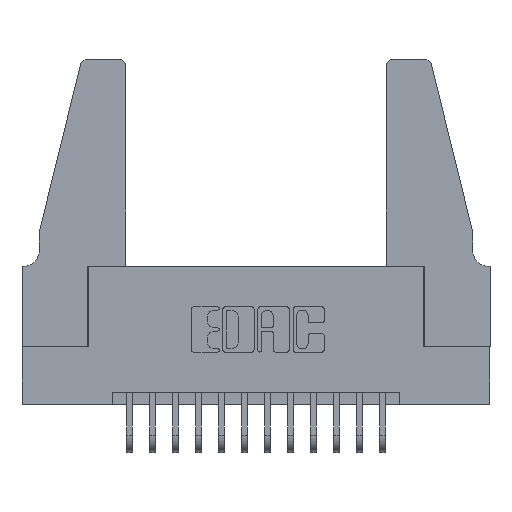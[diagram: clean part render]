
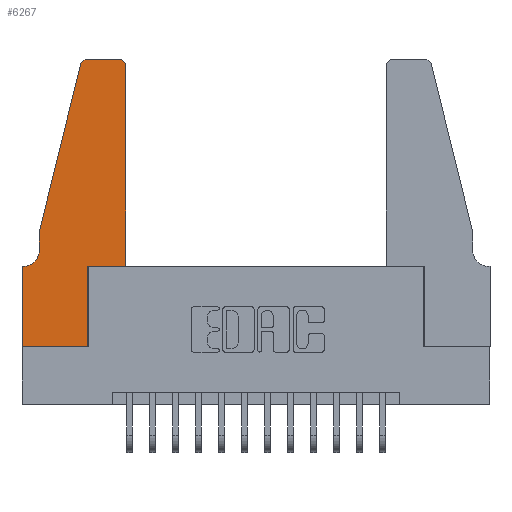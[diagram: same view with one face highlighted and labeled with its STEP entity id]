
A CAD part, top view. The second image highlights one B-rep face of the part: STEP entity #6267.
In plain terms, the highlighted planar face has unit normal (0, 0, 1).
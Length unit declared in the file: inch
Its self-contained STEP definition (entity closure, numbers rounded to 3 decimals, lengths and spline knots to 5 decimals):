
#64 = CARTESIAN_POINT ( 'NONE',  ( 0.2865, 0., 0.37 ) ) ;
#475 = LINE ( 'NONE', #2888, #3563 ) ;
#807 = LINE ( 'NONE', #5140, #5174 ) ;
#1021 = CARTESIAN_POINT ( 'NONE',  ( 0., 0.35, 0.37 ) ) ;
#1147 = EDGE_CURVE ( 'NONE', #10540, #1891, #5495, .T. ) ;
#1408 = CARTESIAN_POINT ( 'NONE',  ( 0.4205, 1.22, 0.37 ) ) ;
#1547 = LINE ( 'NONE', #10497, #8268 ) ;
#1662 = PLANE ( 'NONE',  #8798 ) ;
#1831 = CARTESIAN_POINT ( 'NONE',  ( 0.2605, 1.25, 0.37 ) ) ;
#1891 = VERTEX_POINT ( 'NONE', #16267 ) ;
#2282 = LINE ( 'NONE', #9074, #9048 ) ;
#2426 = VECTOR ( 'NONE', #7248, 39.37008 ) ;
#2433 = ORIENTED_EDGE ( 'NONE', *, *, #2471, .T. ) ;
#2471 = EDGE_CURVE ( 'NONE', #14833, #7350, #475, .T. ) ;
#2714 = DIRECTION ( 'NONE',  ( 1., 0., 0. ) ) ;
#2852 = LINE ( 'NONE', #1831, #2426 ) ;
#2888 = CARTESIAN_POINT ( 'NONE',  ( 0., 0., 0.37 ) ) ;
#2909 = VECTOR ( 'NONE', #13782, 39.37008 ) ;
#3034 = VERTEX_POINT ( 'NONE', #13434 ) ;
#3081 = CIRCLE ( 'NONE', #6327, 0.03 ) ;
#3105 = ORIENTED_EDGE ( 'NONE', *, *, #3518, .T. ) ;
#3156 = CARTESIAN_POINT ( 'NONE',  ( 0.4505, 0.35, 0.37 ) ) ;
#3191 = EDGE_CURVE ( 'NONE', #1891, #4385, #6511, .T. ) ;
#3298 = VERTEX_POINT ( 'NONE', #8658 ) ;
#3370 = VECTOR ( 'NONE', #12187, 39.37008 ) ;
#3416 = EDGE_CURVE ( 'NONE', #3298, #10540, #10298, .T. ) ;
#3518 = EDGE_CURVE ( 'NONE', #7350, #13611, #2282, .T. ) ;
#3563 = VECTOR ( 'NONE', #4241, 39.37008 ) ;
#3834 = DIRECTION ( 'NONE',  ( 0., -1., 0. ) ) ;
#4241 = DIRECTION ( 'NONE',  ( 1., 0., 0. ) ) ;
#4322 = DIRECTION ( 'NONE',  ( 0., 0., 1. ) ) ;
#4385 = VERTEX_POINT ( 'NONE', #8708 ) ;
#4559 = AXIS2_PLACEMENT_3D ( 'NONE', #15573, #7599, #16910 ) ;
#4582 = CIRCLE ( 'NONE', #6427, 0.07 ) ;
#4643 = EDGE_CURVE ( 'NONE', #15009, #15171, #807, .T. ) ;
#5140 = CARTESIAN_POINT ( 'NONE',  ( 0.0755, 0.35, 0.37 ) ) ;
#5162 = DIRECTION ( 'NONE',  ( 0., 0., -1. ) ) ;
#5174 = VECTOR ( 'NONE', #14533, 39.37008 ) ;
#5495 = LINE ( 'NONE', #6586, #3370 ) ;
#5640 = ORIENTED_EDGE ( 'NONE', *, *, #8623, .T. ) ;
#6267 = ADVANCED_FACE ( 'NONE', ( #15178 ), #1662, .T. ) ;
#6327 = AXIS2_PLACEMENT_3D ( 'NONE', #1408, #10789, #2714 ) ;
#6361 = EDGE_CURVE ( 'NONE', #15712, #3298, #2852, .T. ) ;
#6427 = AXIS2_PLACEMENT_3D ( 'NONE', #13206, #5162, #14562 ) ;
#6511 = LINE ( 'NONE', #11110, #2909 ) ;
#6586 = CARTESIAN_POINT ( 'NONE',  ( 0.0755, 0.5, 0.37 ) ) ;
#7248 = DIRECTION ( 'NONE',  ( -1., 0., 0. ) ) ;
#7289 = CARTESIAN_POINT ( 'NONE',  ( 0.4505, 0.35, 0.37 ) ) ;
#7350 = VERTEX_POINT ( 'NONE', #64 ) ;
#7366 = CARTESIAN_POINT ( 'NONE',  ( 0.0055, 0.35, 0.37 ) ) ;
#7599 = DIRECTION ( 'NONE',  ( 0., 0., 1. ) ) ;
#8268 = VECTOR ( 'NONE', #3834, 39.37008 ) ;
#8623 = EDGE_CURVE ( 'NONE', #15171, #14833, #1547, .T. ) ;
#8658 = CARTESIAN_POINT ( 'NONE',  ( 0.284, 1.25, 0.37 ) ) ;
#8708 = CARTESIAN_POINT ( 'NONE',  ( 0.0755, 0.42, 0.37 ) ) ;
#8798 = AXIS2_PLACEMENT_3D ( 'NONE', #12375, #4322, #13709 ) ;
#9048 = VECTOR ( 'NONE', #13074, 39.37008 ) ;
#9074 = CARTESIAN_POINT ( 'NONE',  ( 0.2865, 0.35, 0.37 ) ) ;
#9105 = ORIENTED_EDGE ( 'NONE', *, *, #6361, .T. ) ;
#9597 = LINE ( 'NONE', #7289, #13121 ) ;
#9660 = CARTESIAN_POINT ( 'NONE',  ( 0., 0., 0.37 ) ) ;
#10298 = CIRCLE ( 'NONE', #4559, 0.03 ) ;
#10497 = CARTESIAN_POINT ( 'NONE',  ( 0., 0., 0.37 ) ) ;
#10540 = VERTEX_POINT ( 'NONE', #16713 ) ;
#10789 = DIRECTION ( 'NONE',  ( 0., 0., 1. ) ) ;
#11110 = CARTESIAN_POINT ( 'NONE',  ( 0.0755, 0.5, 0.37 ) ) ;
#11440 = VECTOR ( 'NONE', #12573, 39.37008 ) ;
#12187 = DIRECTION ( 'NONE',  ( -0.239, -0.971, 0. ) ) ;
#12364 = ORIENTED_EDGE ( 'NONE', *, *, #15629, .T. ) ;
#12375 = CARTESIAN_POINT ( 'NONE',  ( 0., 0.35, 0.37 ) ) ;
#12418 = ORIENTED_EDGE ( 'NONE', *, *, #1147, .T. ) ;
#12515 = ORIENTED_EDGE ( 'NONE', *, *, #3416, .T. ) ;
#12573 = DIRECTION ( 'NONE',  ( 1., 0., 0. ) ) ;
#13074 = DIRECTION ( 'NONE',  ( 0., 1., 0. ) ) ;
#13121 = VECTOR ( 'NONE', #16599, 39.37008 ) ;
#13206 = CARTESIAN_POINT ( 'NONE',  ( 0.0055, 0.42, 0.37 ) ) ;
#13221 = EDGE_CURVE ( 'NONE', #4385, #15009, #4582, .T. ) ;
#13307 = ORIENTED_EDGE ( 'NONE', *, *, #4643, .T. ) ;
#13434 = CARTESIAN_POINT ( 'NONE',  ( 0.4505, 0.35, 0.37 ) ) ;
#13435 = ORIENTED_EDGE ( 'NONE', *, *, #16147, .T. ) ;
#13611 = VERTEX_POINT ( 'NONE', #13995 ) ;
#13709 = DIRECTION ( 'NONE',  ( 1., 0., 0. ) ) ;
#13782 = DIRECTION ( 'NONE',  ( 0., -1., 0. ) ) ;
#13995 = CARTESIAN_POINT ( 'NONE',  ( 0.2865, 0.35, 0.37 ) ) ;
#14015 = EDGE_CURVE ( 'NONE', #16557, #15712, #3081, .T. ) ;
#14533 = DIRECTION ( 'NONE',  ( -1., 0., 0. ) ) ;
#14562 = DIRECTION ( 'NONE',  ( -1., 0., 0. ) ) ;
#14592 = ORIENTED_EDGE ( 'NONE', *, *, #14015, .T. ) ;
#14599 = ORIENTED_EDGE ( 'NONE', *, *, #3191, .T. ) ;
#14819 = CARTESIAN_POINT ( 'NONE',  ( 0.4505, 1.22, 0.37 ) ) ;
#14833 = VERTEX_POINT ( 'NONE', #9660 ) ;
#15009 = VERTEX_POINT ( 'NONE', #7366 ) ;
#15171 = VERTEX_POINT ( 'NONE', #1021 ) ;
#15178 = FACE_OUTER_BOUND ( 'NONE', #17099, .T. ) ;
#15387 = LINE ( 'NONE', #3156, #11440 ) ;
#15573 = CARTESIAN_POINT ( 'NONE',  ( 0.284, 1.22, 0.37 ) ) ;
#15629 = EDGE_CURVE ( 'NONE', #3034, #16557, #9597, .T. ) ;
#15712 = VERTEX_POINT ( 'NONE', #16710 ) ;
#16147 = EDGE_CURVE ( 'NONE', #13611, #3034, #15387, .T. ) ;
#16267 = CARTESIAN_POINT ( 'NONE',  ( 0.0755, 0.5, 0.37 ) ) ;
#16456 = ORIENTED_EDGE ( 'NONE', *, *, #13221, .T. ) ;
#16557 = VERTEX_POINT ( 'NONE', #14819 ) ;
#16599 = DIRECTION ( 'NONE',  ( 0., 1., 0. ) ) ;
#16710 = CARTESIAN_POINT ( 'NONE',  ( 0.4205, 1.25, 0.37 ) ) ;
#16713 = CARTESIAN_POINT ( 'NONE',  ( 0.25487, 1.22718, 0.37 ) ) ;
#16910 = DIRECTION ( 'NONE',  ( 1., 0., 0. ) ) ;
#17099 = EDGE_LOOP ( 'NONE', ( #9105, #12515, #12418, #14599, #16456, #13307, #5640, #2433, #3105, #13435, #12364, #14592 ) ) ;
